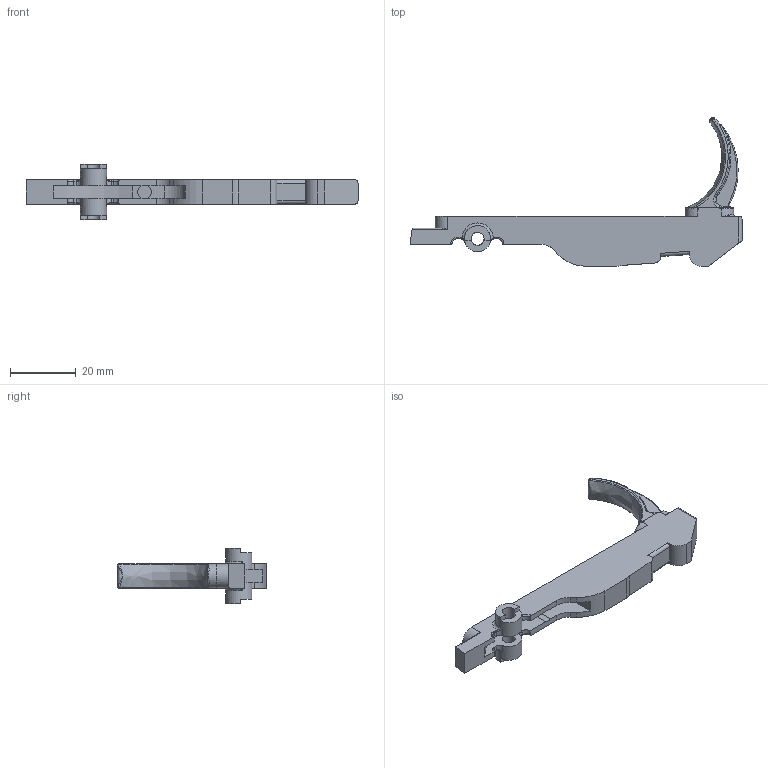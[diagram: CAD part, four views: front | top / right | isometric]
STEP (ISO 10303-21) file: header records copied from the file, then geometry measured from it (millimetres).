
FILE_DESCRIPTION(/* description */ (''),/* implementation_level */ '2;1');
FILE_NAME(/* name */ 'LongTrigger-Curved.step',/* time_stamp */ '2020-10-31T22:00:35-04:00',/* author */ (''),/* organization */ (''),/* preprocessor_version */ 'ST-DEVELOPER v18.1',/* originating_system */ 'Autodesk Translation Framework v9.3.0.1241',/* authorisation */ '');
FILE_SCHEMA (('AUTOMOTIVE_DESIGN { 1 0 10303 214 3 1 1 }'));
Length unit declared in the file: millimetre
Products named in the file (1): LongTrigger
Bounding box: 101.01 x 45.22 x 16.87 mm (x, y, z)
Volume: 8561.8 mm3; surface area: 5613.1 mm2
Topology: 2 solids, 2 shells, 184 faces, 504 edges, 311 vertices
Faces by surface type: plane 57, cylinder 54, bspline 39, torus 32, sphere 2
Full cylindrical faces by diameter (mm): 3.962 x2, 4.216 x1, 7.986 x2
Entity records: 15941 total; most frequent: CARTESIAN_POINT 11484, ORIENTED_EDGE 986, DIRECTION 884, EDGE_CURVE 493, AXIS2_PLACEMENT_3D 345, VERTEX_POINT 311, LINE 194, VECTOR 194
